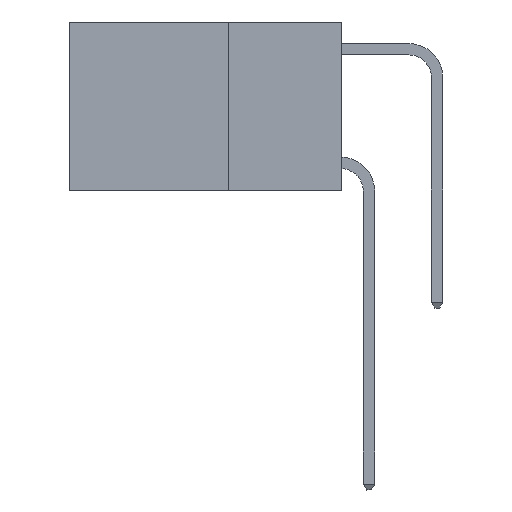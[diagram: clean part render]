
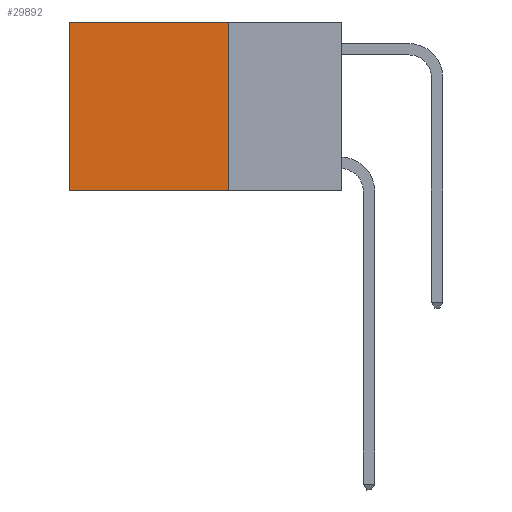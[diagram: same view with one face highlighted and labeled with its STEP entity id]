
A CAD part, left-side view. The second image highlights one B-rep face of the part: STEP entity #29892.
In plain terms, the highlighted planar face has unit normal (-1, 0, 0).
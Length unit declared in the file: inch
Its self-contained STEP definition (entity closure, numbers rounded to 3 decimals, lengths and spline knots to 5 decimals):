
#103 = VERTEX_POINT ( 'NONE', #18027 ) ;
#156 = VECTOR ( 'NONE', #6072, 39.37008 ) ;
#513 = VECTOR ( 'NONE', #11407, 39.37008 ) ;
#792 = EDGE_LOOP ( 'NONE', ( #27652, #28028, #2546, #21500 ) ) ;
#2546 = ORIENTED_EDGE ( 'NONE', *, *, #2847, .F. ) ;
#2847 = EDGE_CURVE ( 'NONE', #3288, #13568, #31057, .T. ) ;
#3245 = CARTESIAN_POINT ( 'NONE',  ( 0.2625, 0.25, 0. ) ) ;
#3288 = VERTEX_POINT ( 'NONE', #3245 ) ;
#4555 = PLANE ( 'NONE',  #5962 ) ;
#5962 = AXIS2_PLACEMENT_3D ( 'NONE', #19745, #22347, #7113 ) ;
#6072 = DIRECTION ( 'NONE',  ( 0., 1., 0. ) ) ;
#6191 = DIRECTION ( 'NONE',  ( 0., 0., -1. ) ) ;
#6389 = VERTEX_POINT ( 'NONE', #12046 ) ;
#7113 = DIRECTION ( 'NONE',  ( 0., 0., -1. ) ) ;
#7200 = CARTESIAN_POINT ( 'NONE',  ( 0.2625, 0.25, -0.37 ) ) ;
#8374 = EDGE_CURVE ( 'NONE', #13568, #6389, #20431, .T. ) ;
#9158 = CARTESIAN_POINT ( 'NONE',  ( 0.2625, 0.25, 0. ) ) ;
#11407 = DIRECTION ( 'NONE',  ( 0., 1., 0. ) ) ;
#12046 = CARTESIAN_POINT ( 'NONE',  ( 0.2625, 0.6, -0.37 ) ) ;
#12428 = LINE ( 'NONE', #26741, #513 ) ;
#13310 = EDGE_CURVE ( 'NONE', #103, #6389, #22168, .T. ) ;
#13568 = VERTEX_POINT ( 'NONE', #7200 ) ;
#14702 = EDGE_CURVE ( 'NONE', #3288, #103, #12428, .T. ) ;
#15336 = VECTOR ( 'NONE', #6191, 39.37008 ) ;
#16289 = CARTESIAN_POINT ( 'NONE',  ( 0.2625, 0.6, 0. ) ) ;
#16523 = FACE_OUTER_BOUND ( 'NONE', #792, .T. ) ;
#18027 = CARTESIAN_POINT ( 'NONE',  ( 0.2625, 0.6, 0. ) ) ;
#18615 = CARTESIAN_POINT ( 'NONE',  ( 0.2625, 0.25, -0.37 ) ) ;
#19047 = VECTOR ( 'NONE', #27011, 39.37008 ) ;
#19745 = CARTESIAN_POINT ( 'NONE',  ( 0.2625, 0.25, 0. ) ) ;
#20431 = LINE ( 'NONE', #18615, #156 ) ;
#21500 = ORIENTED_EDGE ( 'NONE', *, *, #14702, .T. ) ;
#22168 = LINE ( 'NONE', #16289, #15336 ) ;
#22347 = DIRECTION ( 'NONE',  ( 1., 0., 0. ) ) ;
#26741 = CARTESIAN_POINT ( 'NONE',  ( 0.2625, 0.25, 0. ) ) ;
#27011 = DIRECTION ( 'NONE',  ( 0., 0., -1. ) ) ;
#27652 = ORIENTED_EDGE ( 'NONE', *, *, #13310, .T. ) ;
#28028 = ORIENTED_EDGE ( 'NONE', *, *, #8374, .F. ) ;
#29892 = ADVANCED_FACE ( 'NONE', ( #16523 ), #4555, .F. ) ;
#31057 = LINE ( 'NONE', #9158, #19047 ) ;
